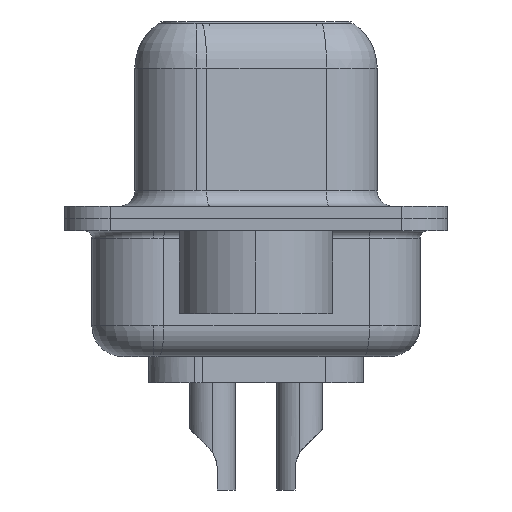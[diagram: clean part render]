
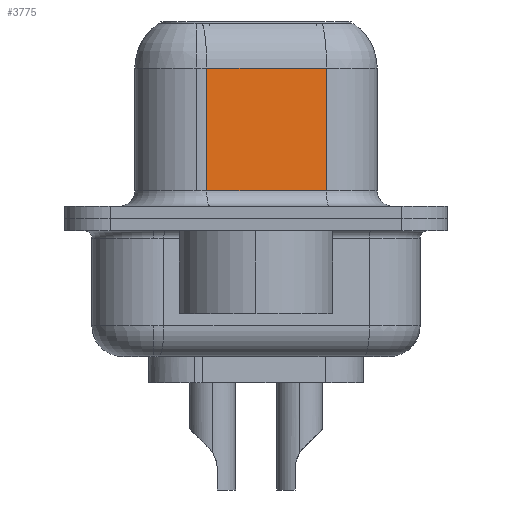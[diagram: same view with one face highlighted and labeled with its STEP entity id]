
A CAD part, left-side view. The second image highlights one B-rep face of the part: STEP entity #3775.
In plain terms, the highlighted planar face has unit normal (-0.985, -0.174, 0).
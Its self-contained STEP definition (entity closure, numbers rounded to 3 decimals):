
#148 = ORIENTED_EDGE ( 'NONE', *, *, #7091, .T. ) ;
#2242 = CARTESIAN_POINT ( 'NONE',  ( 5.068, -2.297, 6.65 ) ) ;
#2667 = DIRECTION ( 'NONE',  ( 0.985, 0.174, 0. ) ) ;
#2740 = ORIENTED_EDGE ( 'NONE', *, *, #9828, .F. ) ;
#3103 = CARTESIAN_POINT ( 'NONE',  ( 4.38, 1.603, 0.9 ) ) ;
#3142 = VERTEX_POINT ( 'NONE', #12919 ) ;
#3240 = VERTEX_POINT ( 'NONE', #8910 ) ;
#3654 = VERTEX_POINT ( 'NONE', #9882 ) ;
#3775 = ADVANCED_FACE ( 'NONE', ( #9251 ), #11803, .F. ) ;
#4141 = ORIENTED_EDGE ( 'NONE', *, *, #7363, .T. ) ;
#5097 = DIRECTION ( 'NONE',  ( 0., 0., -1. ) ) ;
#5716 = VECTOR ( 'NONE', #5097, 1000. ) ;
#5981 = VECTOR ( 'NONE', #18015, 1000. ) ;
#6679 = ORIENTED_EDGE ( 'NONE', *, *, #13886, .T. ) ;
#6907 = LINE ( 'NONE', #8449, #5981 ) ;
#7091 = EDGE_CURVE ( 'NONE', #3654, #16390, #16481, .T. ) ;
#7363 = EDGE_CURVE ( 'NONE', #16390, #3142, #6907, .T. ) ;
#8449 = CARTESIAN_POINT ( 'NONE',  ( 5.068, -2.297, 0.9 ) ) ;
#8910 = CARTESIAN_POINT ( 'NONE',  ( 5.068, -2.297, 4.9 ) ) ;
#9251 = FACE_OUTER_BOUND ( 'NONE', #14214, .T. ) ;
#9270 = LINE ( 'NONE', #12194, #11359 ) ;
#9580 = DIRECTION ( 'NONE',  ( -0.174, 0.985, 0. ) ) ;
#9828 = EDGE_CURVE ( 'NONE', #3240, #3142, #9270, .T. ) ;
#9882 = CARTESIAN_POINT ( 'NONE',  ( 4.38, 1.603, 4.9 ) ) ;
#11116 = CARTESIAN_POINT ( 'NONE',  ( 5.068, -2.297, 4.9 ) ) ;
#11296 = LINE ( 'NONE', #11116, #13779 ) ;
#11359 = VECTOR ( 'NONE', #12108, 1000. ) ;
#11803 = PLANE ( 'NONE',  #12299 ) ;
#12108 = DIRECTION ( 'NONE',  ( 0., 0., -1. ) ) ;
#12194 = CARTESIAN_POINT ( 'NONE',  ( 5.068, -2.297, 6.65 ) ) ;
#12299 = AXIS2_PLACEMENT_3D ( 'NONE', #2242, #2667, #9580 ) ;
#12919 = CARTESIAN_POINT ( 'NONE',  ( 5.068, -2.297, 0.9 ) ) ;
#13575 = CARTESIAN_POINT ( 'NONE',  ( 4.38, 1.603, 6.65 ) ) ;
#13779 = VECTOR ( 'NONE', #15762, 1000. ) ;
#13886 = EDGE_CURVE ( 'NONE', #3240, #3654, #11296, .T. ) ;
#14214 = EDGE_LOOP ( 'NONE', ( #2740, #6679, #148, #4141 ) ) ;
#15762 = DIRECTION ( 'NONE',  ( -0.174, 0.985, 0. ) ) ;
#16390 = VERTEX_POINT ( 'NONE', #3103 ) ;
#16481 = LINE ( 'NONE', #13575, #5716 ) ;
#18015 = DIRECTION ( 'NONE',  ( 0.174, -0.985, 0. ) ) ;
